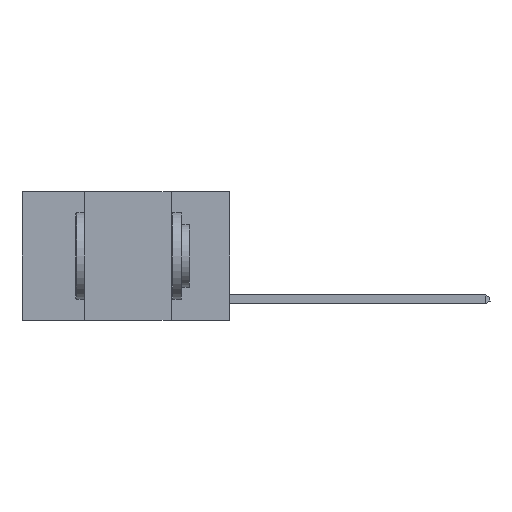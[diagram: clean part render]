
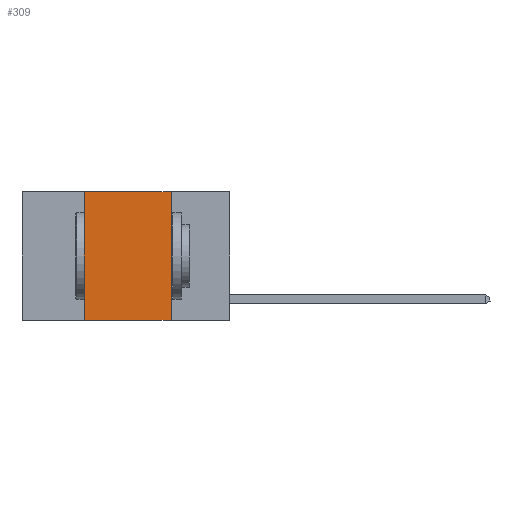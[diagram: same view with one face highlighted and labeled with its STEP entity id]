
A CAD part, left-side view. The second image highlights one B-rep face of the part: STEP entity #309.
In plain terms, the highlighted planar face has unit normal (-1, 0, 0).
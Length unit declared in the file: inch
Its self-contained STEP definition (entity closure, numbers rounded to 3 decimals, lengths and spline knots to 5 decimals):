
#139 = EDGE_CURVE ( 'NONE', #3430, #1800, #9539, .T. ) ;
#277 = FACE_OUTER_BOUND ( 'NONE', #9695, .T. ) ;
#309 = ADVANCED_FACE ( 'NONE', ( #277 ), #3577, .F. ) ;
#324 = DIRECTION ( 'NONE',  ( 0., -1., 0. ) ) ;
#342 = EDGE_CURVE ( 'NONE', #9803, #3430, #7694, .T. ) ;
#467 = ORIENTED_EDGE ( 'NONE', *, *, #10588, .T. ) ;
#1033 = CARTESIAN_POINT ( 'NONE',  ( 0., 0.17, 0. ) ) ;
#1520 = VERTEX_POINT ( 'NONE', #6308 ) ;
#1752 = VECTOR ( 'NONE', #2266, 39.37008 ) ;
#1800 = VERTEX_POINT ( 'NONE', #1033 ) ;
#1805 = DIRECTION ( 'NONE',  ( 0., 0., -1. ) ) ;
#1843 = ORIENTED_EDGE ( 'NONE', *, *, #2013, .F. ) ;
#2013 = EDGE_CURVE ( 'NONE', #1800, #1520, #9962, .T. ) ;
#2266 = DIRECTION ( 'NONE',  ( 0., -1., 0. ) ) ;
#2762 = CARTESIAN_POINT ( 'NONE',  ( 0., 0.6, 0. ) ) ;
#3125 = ORIENTED_EDGE ( 'NONE', *, *, #139, .F. ) ;
#3231 = CARTESIAN_POINT ( 'NONE',  ( 0., 0.6, -0.37 ) ) ;
#3430 = VERTEX_POINT ( 'NONE', #10226 ) ;
#3478 = DIRECTION ( 'NONE',  ( 0., 0., 1. ) ) ;
#3566 = CARTESIAN_POINT ( 'NONE',  ( 0., 0.6, 0. ) ) ;
#3577 = PLANE ( 'NONE',  #6594 ) ;
#4069 = DIRECTION ( 'NONE',  ( 0., 0., -1. ) ) ;
#5148 = CARTESIAN_POINT ( 'NONE',  ( 0., 0.42, -0.37 ) ) ;
#5811 = CARTESIAN_POINT ( 'NONE',  ( 0., 0.17, 0. ) ) ;
#5911 = VECTOR ( 'NONE', #4069, 39.37008 ) ;
#6033 = VECTOR ( 'NONE', #324, 39.37008 ) ;
#6087 = CARTESIAN_POINT ( 'NONE',  ( 0., 0.42, 0. ) ) ;
#6308 = CARTESIAN_POINT ( 'NONE',  ( 0., 0.17, -0.37 ) ) ;
#6594 = AXIS2_PLACEMENT_3D ( 'NONE', #2762, #9237, #1805 ) ;
#7382 = LINE ( 'NONE', #3231, #1752 ) ;
#7694 = LINE ( 'NONE', #6087, #10616 ) ;
#9237 = DIRECTION ( 'NONE',  ( 1., 0., 0. ) ) ;
#9539 = LINE ( 'NONE', #3566, #6033 ) ;
#9695 = EDGE_LOOP ( 'NONE', ( #1843, #3125, #10764, #467 ) ) ;
#9803 = VERTEX_POINT ( 'NONE', #5148 ) ;
#9962 = LINE ( 'NONE', #5811, #5911 ) ;
#10226 = CARTESIAN_POINT ( 'NONE',  ( 0., 0.42, 0. ) ) ;
#10588 = EDGE_CURVE ( 'NONE', #9803, #1520, #7382, .T. ) ;
#10616 = VECTOR ( 'NONE', #3478, 39.37008 ) ;
#10764 = ORIENTED_EDGE ( 'NONE', *, *, #342, .F. ) ;
